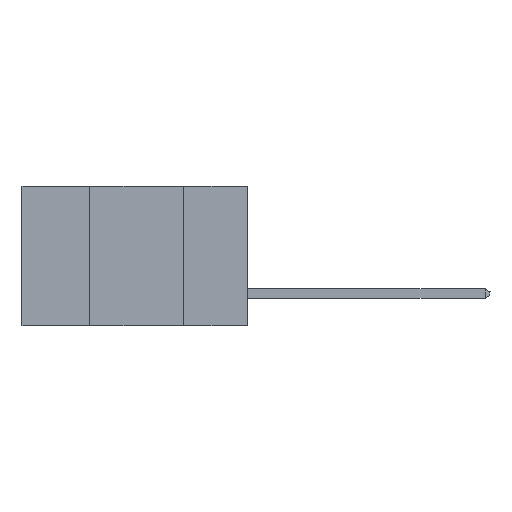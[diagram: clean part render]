
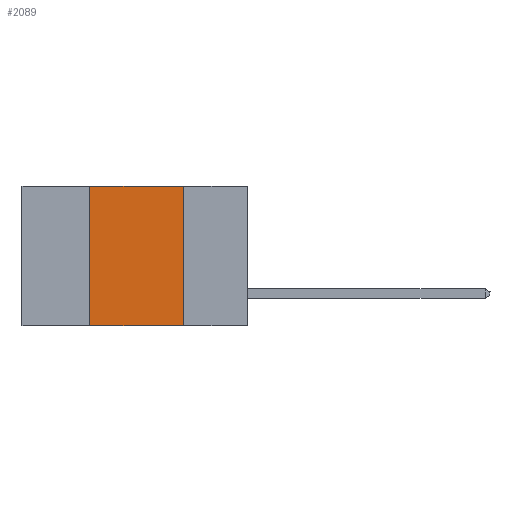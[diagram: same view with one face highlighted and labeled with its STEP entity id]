
A CAD part, left-side view. The second image highlights one B-rep face of the part: STEP entity #2089.
In plain terms, the highlighted planar face has unit normal (-1, 0, 0).
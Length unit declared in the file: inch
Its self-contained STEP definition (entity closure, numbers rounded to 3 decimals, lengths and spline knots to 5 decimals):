
#410 = VECTOR ( 'NONE', #21447, 39.37008 ) ;
#884 = PLANE ( 'NONE',  #11438 ) ;
#1370 = DIRECTION ( 'NONE',  ( 0., 0., 1. ) ) ;
#1558 = DIRECTION ( 'NONE',  ( 0., -1., 0. ) ) ;
#2089 = ADVANCED_FACE ( 'NONE', ( #15795 ), #884, .F. ) ;
#2092 = ORIENTED_EDGE ( 'NONE', *, *, #4553, .F. ) ;
#4553 = EDGE_CURVE ( 'NONE', #16853, #10556, #6370, .T. ) ;
#5355 = EDGE_CURVE ( 'NONE', #18572, #17747, #18319, .T. ) ;
#6370 = LINE ( 'NONE', #16813, #16012 ) ;
#6845 = EDGE_LOOP ( 'NONE', ( #11988, #2092, #11361, #10395 ) ) ;
#7642 = VECTOR ( 'NONE', #19557, 39.37008 ) ;
#7688 = DIRECTION ( 'NONE',  ( 1., 0., 0. ) ) ;
#9220 = LINE ( 'NONE', #19779, #7642 ) ;
#10395 = ORIENTED_EDGE ( 'NONE', *, *, #5355, .T. ) ;
#10425 = CARTESIAN_POINT ( 'NONE',  ( 0., 0.42, -0.37 ) ) ;
#10556 = VERTEX_POINT ( 'NONE', #14157 ) ;
#11361 = ORIENTED_EDGE ( 'NONE', *, *, #15923, .F. ) ;
#11438 = AXIS2_PLACEMENT_3D ( 'NONE', #21134, #7688, #15906 ) ;
#11988 = ORIENTED_EDGE ( 'NONE', *, *, #18297, .F. ) ;
#13216 = CARTESIAN_POINT ( 'NONE',  ( 0., 0.42, 0. ) ) ;
#14157 = CARTESIAN_POINT ( 'NONE',  ( 0., 0.17, 0. ) ) ;
#14936 = LINE ( 'NONE', #16837, #18730 ) ;
#15795 = FACE_OUTER_BOUND ( 'NONE', #6845, .T. ) ;
#15906 = DIRECTION ( 'NONE',  ( 0., 0., -1. ) ) ;
#15923 = EDGE_CURVE ( 'NONE', #18572, #16853, #14936, .T. ) ;
#16012 = VECTOR ( 'NONE', #1558, 39.37008 ) ;
#16547 = CARTESIAN_POINT ( 'NONE',  ( 0., 0.6, -0.37 ) ) ;
#16813 = CARTESIAN_POINT ( 'NONE',  ( 0., 0.6, 0. ) ) ;
#16837 = CARTESIAN_POINT ( 'NONE',  ( 0., 0.42, -0.37 ) ) ;
#16853 = VERTEX_POINT ( 'NONE', #13216 ) ;
#17747 = VERTEX_POINT ( 'NONE', #20921 ) ;
#18297 = EDGE_CURVE ( 'NONE', #10556, #17747, #9220, .T. ) ;
#18319 = LINE ( 'NONE', #16547, #410 ) ;
#18572 = VERTEX_POINT ( 'NONE', #10425 ) ;
#18730 = VECTOR ( 'NONE', #1370, 39.37008 ) ;
#19557 = DIRECTION ( 'NONE',  ( 0., 0., -1. ) ) ;
#19779 = CARTESIAN_POINT ( 'NONE',  ( 0., 0.17, -0.37 ) ) ;
#20921 = CARTESIAN_POINT ( 'NONE',  ( 0., 0.17, -0.37 ) ) ;
#21134 = CARTESIAN_POINT ( 'NONE',  ( 0., 0.6, 0. ) ) ;
#21447 = DIRECTION ( 'NONE',  ( 0., -1., 0. ) ) ;
